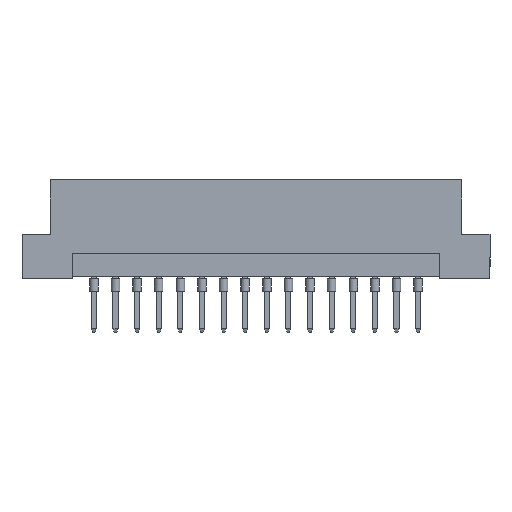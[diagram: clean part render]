
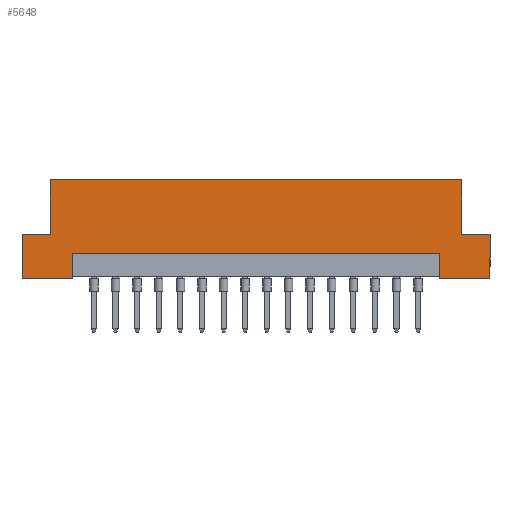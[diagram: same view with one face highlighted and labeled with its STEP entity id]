
A CAD part, front view. The second image highlights one B-rep face of the part: STEP entity #5648.
In plain terms, the highlighted planar face has unit normal (0, -1, 0).
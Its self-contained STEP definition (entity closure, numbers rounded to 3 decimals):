
#131 = CARTESIAN_POINT ( 'NONE',  ( -21.6, -4.3, 0. ) ) ;
#210 = CARTESIAN_POINT ( 'NONE',  ( -27.5, -4.3, 5.2 ) ) ;
#226 = DIRECTION ( 'NONE',  ( 0., 1., 0. ) ) ;
#241 = EDGE_CURVE ( 'NONE', #6538, #6390, #2988, .T. ) ;
#255 = CARTESIAN_POINT ( 'NONE',  ( 21.6, -4.3, 0. ) ) ;
#265 = CARTESIAN_POINT ( 'NONE',  ( -24.2, -4.3, 5.2 ) ) ;
#326 = VECTOR ( 'NONE', #5216, 1000. ) ;
#416 = DIRECTION ( 'NONE',  ( 0., 0., 1. ) ) ;
#428 = VECTOR ( 'NONE', #1411, 1000. ) ;
#436 = ORIENTED_EDGE ( 'NONE', *, *, #3131, .T. ) ;
#463 = CARTESIAN_POINT ( 'NONE',  ( -21.6, -4.3, 3. ) ) ;
#466 = EDGE_CURVE ( 'NONE', #1225, #3252, #1210, .T. ) ;
#503 = CARTESIAN_POINT ( 'NONE',  ( -27.5, -4.3, 11.6 ) ) ;
#557 = CARTESIAN_POINT ( 'NONE',  ( -21.6, -4.3, 0.2 ) ) ;
#838 = DIRECTION ( 'NONE',  ( 1., 0., 0. ) ) ;
#929 = LINE ( 'NONE', #265, #428 ) ;
#938 = ORIENTED_EDGE ( 'NONE', *, *, #960, .F. ) ;
#960 = EDGE_CURVE ( 'NONE', #7161, #2780, #5093, .T. ) ;
#990 = CARTESIAN_POINT ( 'NONE',  ( -24.2, -4.3, 11.6 ) ) ;
#1210 = LINE ( 'NONE', #557, #3922 ) ;
#1225 = VERTEX_POINT ( 'NONE', #2491 ) ;
#1257 = VECTOR ( 'NONE', #4460, 1000. ) ;
#1331 = PLANE ( 'NONE',  #5184 ) ;
#1347 = DIRECTION ( 'NONE',  ( 1., 0., 0. ) ) ;
#1370 = EDGE_CURVE ( 'NONE', #1225, #6547, #1667, .T. ) ;
#1411 = DIRECTION ( 'NONE',  ( 0., 0., 1. ) ) ;
#1432 = VECTOR ( 'NONE', #6695, 1000. ) ;
#1433 = FACE_OUTER_BOUND ( 'NONE', #3113, .T. ) ;
#1498 = ORIENTED_EDGE ( 'NONE', *, *, #5132, .F. ) ;
#1515 = ORIENTED_EDGE ( 'NONE', *, *, #1370, .T. ) ;
#1667 = LINE ( 'NONE', #463, #1257 ) ;
#1696 = LINE ( 'NONE', #7059, #7163 ) ;
#1714 = EDGE_CURVE ( 'NONE', #5741, #2780, #1696, .T. ) ;
#1827 = CARTESIAN_POINT ( 'NONE',  ( 27.5, -4.3, 0. ) ) ;
#1939 = EDGE_CURVE ( 'NONE', #6954, #3070, #6222, .T. ) ;
#2087 = CARTESIAN_POINT ( 'NONE',  ( 24.2, -4.3, 11.6 ) ) ;
#2491 = CARTESIAN_POINT ( 'NONE',  ( -21.6, -4.3, 3. ) ) ;
#2577 = LINE ( 'NONE', #7150, #4022 ) ;
#2598 = CARTESIAN_POINT ( 'NONE',  ( 21.6, -4.3, 0.2 ) ) ;
#2780 = VERTEX_POINT ( 'NONE', #2087 ) ;
#2885 = ORIENTED_EDGE ( 'NONE', *, *, #4429, .F. ) ;
#2988 = LINE ( 'NONE', #5252, #326 ) ;
#3006 = VECTOR ( 'NONE', #1347, 1000. ) ;
#3007 = CARTESIAN_POINT ( 'NONE',  ( 21.6, -4.3, 3. ) ) ;
#3070 = VERTEX_POINT ( 'NONE', #3224 ) ;
#3113 = EDGE_LOOP ( 'NONE', ( #1515, #7021, #5123, #2885, #4808, #3500, #938, #1498, #4990, #436, #6996, #6818 ) ) ;
#3131 = EDGE_CURVE ( 'NONE', #6538, #3530, #7070, .T. ) ;
#3224 = CARTESIAN_POINT ( 'NONE',  ( 27.5, -4.3, 0. ) ) ;
#3252 = VERTEX_POINT ( 'NONE', #131 ) ;
#3255 = VERTEX_POINT ( 'NONE', #6129 ) ;
#3257 = DIRECTION ( 'NONE',  ( 0., 0., -1. ) ) ;
#3473 = CARTESIAN_POINT ( 'NONE',  ( 27.5, -4.3, 11.6 ) ) ;
#3500 = ORIENTED_EDGE ( 'NONE', *, *, #1714, .T. ) ;
#3529 = EDGE_CURVE ( 'NONE', #6954, #6547, #4937, .T. ) ;
#3530 = VERTEX_POINT ( 'NONE', #4861 ) ;
#3922 = VECTOR ( 'NONE', #6717, 1000. ) ;
#3951 = CARTESIAN_POINT ( 'NONE',  ( -24.2, -4.3, 5.2 ) ) ;
#4022 = VECTOR ( 'NONE', #5026, 1000. ) ;
#4121 = CARTESIAN_POINT ( 'NONE',  ( 27.5, -4.3, 11.6 ) ) ;
#4363 = CARTESIAN_POINT ( 'NONE',  ( 24.2, -4.3, 5.2 ) ) ;
#4429 = EDGE_CURVE ( 'NONE', #3255, #3070, #2577, .T. ) ;
#4460 = DIRECTION ( 'NONE',  ( 1., 0., 0. ) ) ;
#4593 = CARTESIAN_POINT ( 'NONE',  ( 27.5, -4.3, 0. ) ) ;
#4808 = ORIENTED_EDGE ( 'NONE', *, *, #6032, .F. ) ;
#4861 = CARTESIAN_POINT ( 'NONE',  ( -27.5, -4.3, 0. ) ) ;
#4937 = LINE ( 'NONE', #2598, #6591 ) ;
#4975 = DIRECTION ( 'NONE',  ( 0., 0., 1. ) ) ;
#4990 = ORIENTED_EDGE ( 'NONE', *, *, #241, .F. ) ;
#5026 = DIRECTION ( 'NONE',  ( 0., 0., -1. ) ) ;
#5093 = LINE ( 'NONE', #3473, #3006 ) ;
#5123 = ORIENTED_EDGE ( 'NONE', *, *, #1939, .T. ) ;
#5132 = EDGE_CURVE ( 'NONE', #6390, #7161, #929, .T. ) ;
#5184 = AXIS2_PLACEMENT_3D ( 'NONE', #4121, #226, #6323 ) ;
#5216 = DIRECTION ( 'NONE',  ( 1., 0., 0. ) ) ;
#5252 = CARTESIAN_POINT ( 'NONE',  ( -27.5, -4.3, 5.2 ) ) ;
#5296 = VECTOR ( 'NONE', #838, 1000. ) ;
#5599 = DIRECTION ( 'NONE',  ( 1., 0., 0. ) ) ;
#5648 = ADVANCED_FACE ( 'NONE', ( #1433 ), #1331, .F. ) ;
#5741 = VERTEX_POINT ( 'NONE', #4363 ) ;
#5852 = CARTESIAN_POINT ( 'NONE',  ( 27.5, -4.3, 5.2 ) ) ;
#6004 = VECTOR ( 'NONE', #3257, 1000. ) ;
#6032 = EDGE_CURVE ( 'NONE', #5741, #3255, #6384, .T. ) ;
#6129 = CARTESIAN_POINT ( 'NONE',  ( 27.5, -4.3, 5.2 ) ) ;
#6178 = LINE ( 'NONE', #1827, #6539 ) ;
#6222 = LINE ( 'NONE', #4593, #1432 ) ;
#6323 = DIRECTION ( 'NONE',  ( -1., 0., 0. ) ) ;
#6384 = LINE ( 'NONE', #5852, #5296 ) ;
#6390 = VERTEX_POINT ( 'NONE', #3951 ) ;
#6538 = VERTEX_POINT ( 'NONE', #210 ) ;
#6539 = VECTOR ( 'NONE', #5599, 1000. ) ;
#6547 = VERTEX_POINT ( 'NONE', #3007 ) ;
#6591 = VECTOR ( 'NONE', #4975, 1000. ) ;
#6695 = DIRECTION ( 'NONE',  ( 1., 0., 0. ) ) ;
#6717 = DIRECTION ( 'NONE',  ( 0., 0., -1. ) ) ;
#6800 = EDGE_CURVE ( 'NONE', #3530, #3252, #6178, .T. ) ;
#6818 = ORIENTED_EDGE ( 'NONE', *, *, #466, .F. ) ;
#6954 = VERTEX_POINT ( 'NONE', #255 ) ;
#6996 = ORIENTED_EDGE ( 'NONE', *, *, #6800, .T. ) ;
#7021 = ORIENTED_EDGE ( 'NONE', *, *, #3529, .F. ) ;
#7059 = CARTESIAN_POINT ( 'NONE',  ( 24.2, -4.3, 5.2 ) ) ;
#7070 = LINE ( 'NONE', #503, #6004 ) ;
#7150 = CARTESIAN_POINT ( 'NONE',  ( 27.5, -4.3, 11.6 ) ) ;
#7161 = VERTEX_POINT ( 'NONE', #990 ) ;
#7163 = VECTOR ( 'NONE', #416, 1000. ) ;
